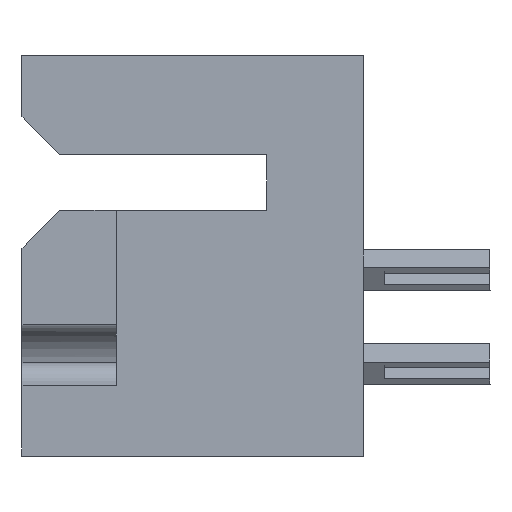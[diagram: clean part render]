
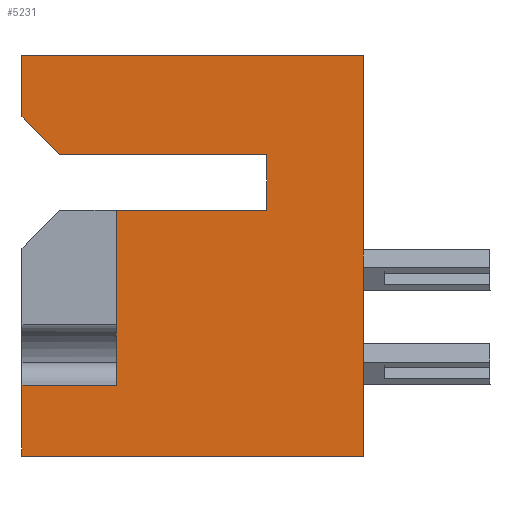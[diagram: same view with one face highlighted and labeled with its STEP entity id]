
A CAD part, left-side view. The second image highlights one B-rep face of the part: STEP entity #5231.
In plain terms, the highlighted planar face has unit normal (-1, 0, 0).
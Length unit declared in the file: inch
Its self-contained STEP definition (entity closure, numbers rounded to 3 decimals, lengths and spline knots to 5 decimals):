
#59 = LINE ( 'NONE', #18703, #3869 ) ;
#258 = CARTESIAN_POINT ( 'NONE',  ( 0., 0.453, -0.437 ) ) ;
#283 = ORIENTED_EDGE ( 'NONE', *, *, #15112, .F. ) ;
#386 = DIRECTION ( 'NONE',  ( 0., 1., 0. ) ) ;
#505 = LINE ( 'NONE', #4848, #8608 ) ;
#533 = ORIENTED_EDGE ( 'NONE', *, *, #13050, .T. ) ;
#634 = VERTEX_POINT ( 'NONE', #12039 ) ;
#974 = ORIENTED_EDGE ( 'NONE', *, *, #20808, .F. ) ;
#1312 = VERTEX_POINT ( 'NONE', #15232 ) ;
#1565 = VERTEX_POINT ( 'NONE', #9912 ) ;
#1635 = CARTESIAN_POINT ( 'NONE',  ( 0., 0.403, -0.131 ) ) ;
#2018 = VERTEX_POINT ( 'NONE', #258 ) ;
#2026 = CARTESIAN_POINT ( 'NONE',  ( 0., 0.128, -0.131 ) ) ;
#2585 = DIRECTION ( 'NONE',  ( 0., 1., 0. ) ) ;
#2619 = LINE ( 'NONE', #3094, #10963 ) ;
#2777 = DIRECTION ( 'NONE',  ( 0., 0., 1. ) ) ;
#3094 = CARTESIAN_POINT ( 'NONE',  ( 0., 0.453, -0.531 ) ) ;
#3363 = DIRECTION ( 'NONE',  ( 0., 0., 1. ) ) ;
#3506 = CARTESIAN_POINT ( 'NONE',  ( 0., 0.453, 0. ) ) ;
#3843 = EDGE_CURVE ( 'NONE', #1565, #13309, #5690, .T. ) ;
#3869 = VECTOR ( 'NONE', #10812, 39.37008 ) ;
#4112 = EDGE_CURVE ( 'NONE', #13309, #634, #15531, .T. ) ;
#4130 = ORIENTED_EDGE ( 'NONE', *, *, #6676, .F. ) ;
#4420 = CARTESIAN_POINT ( 'NONE',  ( 0., 0., 0. ) ) ;
#4453 = LINE ( 'NONE', #6820, #9017 ) ;
#4537 = CARTESIAN_POINT ( 'NONE',  ( 0., 0.328, -0.205 ) ) ;
#4610 = FACE_OUTER_BOUND ( 'NONE', #9891, .T. ) ;
#4848 = CARTESIAN_POINT ( 'NONE',  ( 0., 0.328, -0.205 ) ) ;
#4985 = CARTESIAN_POINT ( 'NONE',  ( 0., 0., 0. ) ) ;
#5005 = VERTEX_POINT ( 'NONE', #12124 ) ;
#5018 = CARTESIAN_POINT ( 'NONE',  ( 0., 0.453, 0. ) ) ;
#5103 = LINE ( 'NONE', #5018, #8395 ) ;
#5231 = ADVANCED_FACE ( 'NONE', ( #4610 ), #5842, .F. ) ;
#5622 = VECTOR ( 'NONE', #3363, 39.37008 ) ;
#5690 = LINE ( 'NONE', #6705, #11987 ) ;
#5842 = PLANE ( 'NONE',  #18601 ) ;
#6285 = ORIENTED_EDGE ( 'NONE', *, *, #9819, .F. ) ;
#6366 = DIRECTION ( 'NONE',  ( 0., -1., 0. ) ) ;
#6460 = DIRECTION ( 'NONE',  ( 0., -0.707, -0.707 ) ) ;
#6578 = VERTEX_POINT ( 'NONE', #4985 ) ;
#6676 = EDGE_CURVE ( 'NONE', #5005, #6887, #505, .T. ) ;
#6705 = CARTESIAN_POINT ( 'NONE',  ( 0., 0.128, -0.131 ) ) ;
#6820 = CARTESIAN_POINT ( 'NONE',  ( 0., 0.128, -0.205 ) ) ;
#6887 = VERTEX_POINT ( 'NONE', #4537 ) ;
#7177 = VERTEX_POINT ( 'NONE', #11321 ) ;
#8143 = VECTOR ( 'NONE', #6460, 39.37008 ) ;
#8395 = VECTOR ( 'NONE', #10061, 39.37008 ) ;
#8559 = ORIENTED_EDGE ( 'NONE', *, *, #4112, .F. ) ;
#8608 = VECTOR ( 'NONE', #12954, 39.37008 ) ;
#8662 = LINE ( 'NONE', #1635, #8143 ) ;
#8996 = EDGE_CURVE ( 'NONE', #12847, #7177, #2619, .T. ) ;
#9017 = VECTOR ( 'NONE', #386, 39.37008 ) ;
#9819 = EDGE_CURVE ( 'NONE', #1312, #12225, #13974, .T. ) ;
#9836 = CARTESIAN_POINT ( 'NONE',  ( 0., 0.453, 0. ) ) ;
#9891 = EDGE_LOOP ( 'NONE', ( #18045, #283, #15544, #10080, #974, #6285, #16945, #8559, #13557, #533, #4130 ) ) ;
#9912 = CARTESIAN_POINT ( 'NONE',  ( 0., 0.128, -0.205 ) ) ;
#10061 = DIRECTION ( 'NONE',  ( 0., 0., 1. ) ) ;
#10080 = ORIENTED_EDGE ( 'NONE', *, *, #18662, .T. ) ;
#10222 = EDGE_CURVE ( 'NONE', #1312, #634, #8662, .T. ) ;
#10665 = DIRECTION ( 'NONE',  ( 0., 0., -1. ) ) ;
#10805 = VECTOR ( 'NONE', #2585, 39.37008 ) ;
#10812 = DIRECTION ( 'NONE',  ( 0., -1., 0. ) ) ;
#10963 = VECTOR ( 'NONE', #6366, 39.37008 ) ;
#11321 = CARTESIAN_POINT ( 'NONE',  ( 0., 0., -0.531 ) ) ;
#11987 = VECTOR ( 'NONE', #19255, 39.37008 ) ;
#12039 = CARTESIAN_POINT ( 'NONE',  ( 0., 0.403, -0.131 ) ) ;
#12093 = DIRECTION ( 'NONE',  ( 1., 0., 0. ) ) ;
#12124 = CARTESIAN_POINT ( 'NONE',  ( 0., 0.328, -0.437 ) ) ;
#12225 = VERTEX_POINT ( 'NONE', #9836 ) ;
#12621 = EDGE_CURVE ( 'NONE', #5005, #2018, #18122, .T. ) ;
#12847 = VERTEX_POINT ( 'NONE', #17623 ) ;
#12954 = DIRECTION ( 'NONE',  ( 0., 0., 1. ) ) ;
#13050 = EDGE_CURVE ( 'NONE', #1565, #6887, #4453, .T. ) ;
#13309 = VERTEX_POINT ( 'NONE', #18731 ) ;
#13557 = ORIENTED_EDGE ( 'NONE', *, *, #3843, .F. ) ;
#13974 = LINE ( 'NONE', #3506, #5622 ) ;
#15031 = VECTOR ( 'NONE', #2777, 39.37008 ) ;
#15112 = EDGE_CURVE ( 'NONE', #12847, #2018, #5103, .T. ) ;
#15232 = CARTESIAN_POINT ( 'NONE',  ( 0., 0.453, -0.081 ) ) ;
#15266 = VECTOR ( 'NONE', #16280, 39.37008 ) ;
#15445 = CARTESIAN_POINT ( 'NONE',  ( 0., 0.328, -0.437 ) ) ;
#15531 = LINE ( 'NONE', #2026, #15266 ) ;
#15544 = ORIENTED_EDGE ( 'NONE', *, *, #8996, .T. ) ;
#16266 = LINE ( 'NONE', #4420, #15031 ) ;
#16280 = DIRECTION ( 'NONE',  ( 0., 1., 0. ) ) ;
#16945 = ORIENTED_EDGE ( 'NONE', *, *, #10222, .T. ) ;
#17263 = CARTESIAN_POINT ( 'NONE',  ( 0., 0.453, 0. ) ) ;
#17623 = CARTESIAN_POINT ( 'NONE',  ( 0., 0.453, -0.531 ) ) ;
#18045 = ORIENTED_EDGE ( 'NONE', *, *, #12621, .T. ) ;
#18122 = LINE ( 'NONE', #15445, #10805 ) ;
#18601 = AXIS2_PLACEMENT_3D ( 'NONE', #17263, #12093, #10665 ) ;
#18662 = EDGE_CURVE ( 'NONE', #7177, #6578, #16266, .T. ) ;
#18703 = CARTESIAN_POINT ( 'NONE',  ( 0., 0.453, 0. ) ) ;
#18731 = CARTESIAN_POINT ( 'NONE',  ( 0., 0.128, -0.131 ) ) ;
#19255 = DIRECTION ( 'NONE',  ( 0., 0., 1. ) ) ;
#20808 = EDGE_CURVE ( 'NONE', #12225, #6578, #59, .T. ) ;
